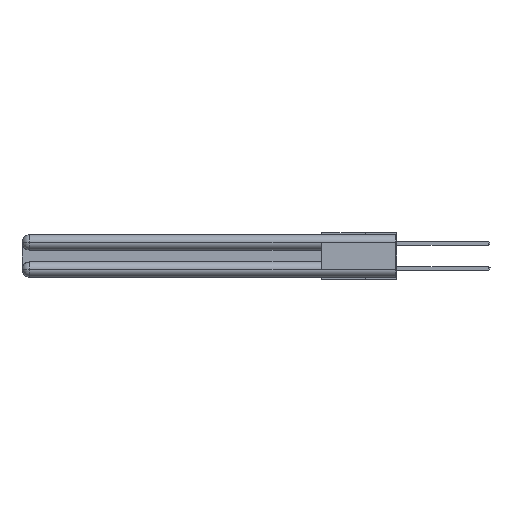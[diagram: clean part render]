
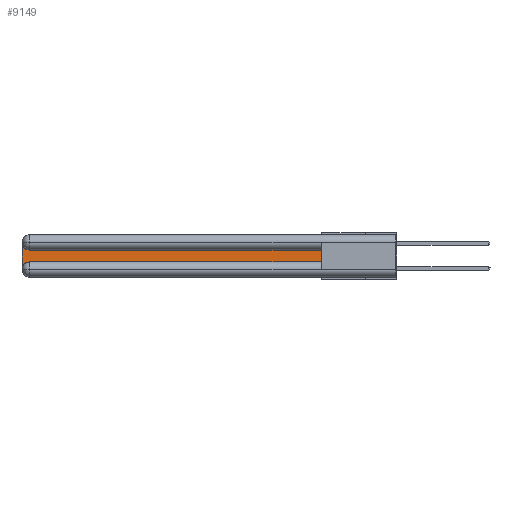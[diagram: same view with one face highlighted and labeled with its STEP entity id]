
A CAD part, left-side view. The second image highlights one B-rep face of the part: STEP entity #9149.
In plain terms, the highlighted planar face has unit normal (-1, 0, 0).
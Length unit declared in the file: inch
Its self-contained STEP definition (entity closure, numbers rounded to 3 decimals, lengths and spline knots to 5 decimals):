
#1332 = LINE ( 'NONE', #15709, #1716 ) ;
#1336 = VECTOR ( 'NONE', #6972, 39.37008 ) ;
#1716 = VECTOR ( 'NONE', #12691, 39.37008 ) ;
#1768 = EDGE_CURVE ( 'NONE', #30197, #10140, #8942, .T. ) ;
#1988 = CARTESIAN_POINT ( 'NONE',  ( 0.075, 0.6, -0.2175 ) ) ;
#4029 = AXIS2_PLACEMENT_3D ( 'NONE', #7597, #22488, #4576 ) ;
#4283 = EDGE_CURVE ( 'NONE', #31926, #7221, #17389, .T. ) ;
#4576 = DIRECTION ( 'NONE',  ( 0., 0., -1. ) ) ;
#4630 = ORIENTED_EDGE ( 'NONE', *, *, #26682, .T. ) ;
#5511 = CARTESIAN_POINT ( 'NONE',  ( 0.075, 0.6, -0.1225 ) ) ;
#6308 = DIRECTION ( 'NONE',  ( 1., 0., 0. ) ) ;
#6417 = DIRECTION ( 'NONE',  ( 0., 0., -1. ) ) ;
#6622 = ORIENTED_EDGE ( 'NONE', *, *, #26098, .T. ) ;
#6771 = VERTEX_POINT ( 'NONE', #20274 ) ;
#6972 = DIRECTION ( 'NONE',  ( 0., 1., 0. ) ) ;
#7221 = VERTEX_POINT ( 'NONE', #8974 ) ;
#7597 = CARTESIAN_POINT ( 'NONE',  ( 0.075, 3., -0.1225 ) ) ;
#8547 = EDGE_CURVE ( 'NONE', #15297, #6771, #27930, .T. ) ;
#8942 = LINE ( 'NONE', #12788, #22161 ) ;
#8974 = CARTESIAN_POINT ( 'NONE',  ( 0.075, 2.94, -0.2175 ) ) ;
#9149 = ADVANCED_FACE ( 'NONE', ( #19521 ), #33071, .F. ) ;
#9218 = CARTESIAN_POINT ( 'NONE',  ( 0.075, 2.94, -0.2775 ) ) ;
#9792 = ORIENTED_EDGE ( 'NONE', *, *, #8547, .T. ) ;
#10140 = VERTEX_POINT ( 'NONE', #5511 ) ;
#11693 = VECTOR ( 'NONE', #32599, 39.37008 ) ;
#12691 = DIRECTION ( 'NONE',  ( 0., 0., -1. ) ) ;
#12788 = CARTESIAN_POINT ( 'NONE',  ( 0.075, 0.6, -0.2175 ) ) ;
#12905 = AXIS2_PLACEMENT_3D ( 'NONE', #9218, #32137, #16835 ) ;
#14509 = LINE ( 'NONE', #27656, #1336 ) ;
#15297 = VERTEX_POINT ( 'NONE', #18972 ) ;
#15709 = CARTESIAN_POINT ( 'NONE',  ( 0.075, 3., -0.2175 ) ) ;
#15991 = ORIENTED_EDGE ( 'NONE', *, *, #4283, .T. ) ;
#16835 = DIRECTION ( 'NONE',  ( 0., 0., -1. ) ) ;
#16844 = ORIENTED_EDGE ( 'NONE', *, *, #19390, .T. ) ;
#17389 = CIRCLE ( 'NONE', #12905, 0.06 ) ;
#17593 = ORIENTED_EDGE ( 'NONE', *, *, #1768, .T. ) ;
#18972 = CARTESIAN_POINT ( 'NONE',  ( 0.075, 2.94, -0.1225 ) ) ;
#19390 = EDGE_CURVE ( 'NONE', #6771, #31926, #1332, .T. ) ;
#19467 = EDGE_LOOP ( 'NONE', ( #6622, #9792, #16844, #15991, #4630, #17593 ) ) ;
#19521 = FACE_OUTER_BOUND ( 'NONE', #19467, .T. ) ;
#20210 = DIRECTION ( 'NONE',  ( 0., 0., 1. ) ) ;
#20274 = CARTESIAN_POINT ( 'NONE',  ( 0.075, 3., -0.0625 ) ) ;
#22161 = VECTOR ( 'NONE', #20210, 39.37008 ) ;
#22488 = DIRECTION ( 'NONE',  ( 1., 0., 0. ) ) ;
#22906 = CARTESIAN_POINT ( 'NONE',  ( 0.075, 0.6, -0.2175 ) ) ;
#24173 = AXIS2_PLACEMENT_3D ( 'NONE', #31543, #6308, #6417 ) ;
#26098 = EDGE_CURVE ( 'NONE', #10140, #15297, #14509, .T. ) ;
#26682 = EDGE_CURVE ( 'NONE', #7221, #30197, #26925, .T. ) ;
#26925 = LINE ( 'NONE', #1988, #11693 ) ;
#27146 = CARTESIAN_POINT ( 'NONE',  ( 0.075, 3., -0.2775 ) ) ;
#27656 = CARTESIAN_POINT ( 'NONE',  ( 0.075, 0.6, -0.1225 ) ) ;
#27930 = CIRCLE ( 'NONE', #24173, 0.06 ) ;
#30197 = VERTEX_POINT ( 'NONE', #22906 ) ;
#31543 = CARTESIAN_POINT ( 'NONE',  ( 0.075, 2.94, -0.0625 ) ) ;
#31926 = VERTEX_POINT ( 'NONE', #27146 ) ;
#32137 = DIRECTION ( 'NONE',  ( 1., 0., 0. ) ) ;
#32599 = DIRECTION ( 'NONE',  ( 0., -1., 0. ) ) ;
#33071 = PLANE ( 'NONE',  #4029 ) ;
